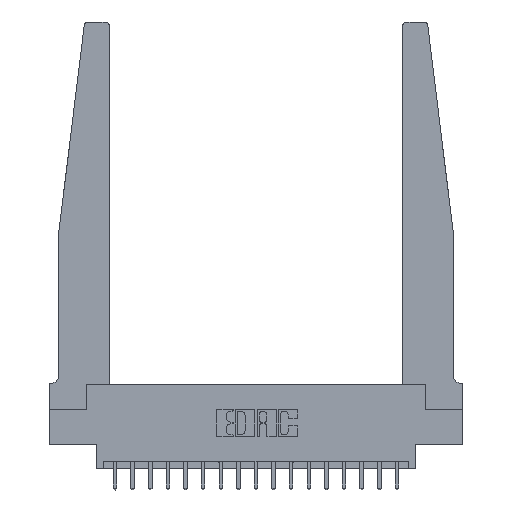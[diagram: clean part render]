
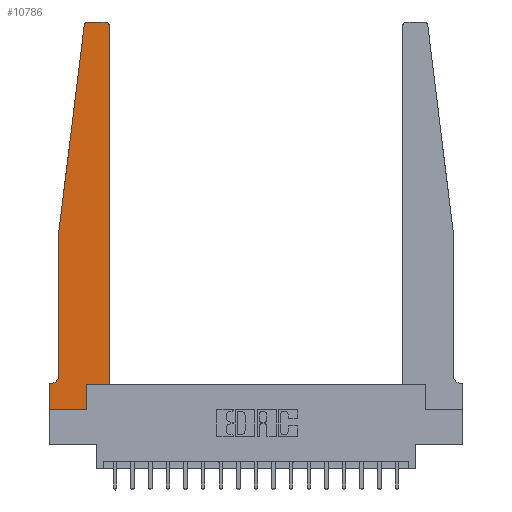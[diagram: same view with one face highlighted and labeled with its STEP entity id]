
A CAD part, top view. The second image highlights one B-rep face of the part: STEP entity #10786.
In plain terms, the highlighted planar face has unit normal (0, 0, 1).
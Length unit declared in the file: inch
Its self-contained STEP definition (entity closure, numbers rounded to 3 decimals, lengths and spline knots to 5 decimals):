
#241 = EDGE_LOOP ( 'NONE', ( #7035, #4532, #2124, #3526, #17690, #8362, #7647, #2840, #19340, #8499, #999, #5198 ) ) ;
#347 = EDGE_CURVE ( 'NONE', #17558, #3035, #9736, .T. ) ;
#404 = VERTEX_POINT ( 'NONE', #5014 ) ;
#543 = DIRECTION ( 'NONE',  ( 1., 0., 0. ) ) ;
#586 = CARTESIAN_POINT ( 'NONE',  ( 0., 0., 0.37 ) ) ;
#904 = FACE_OUTER_BOUND ( 'NONE', #241, .T. ) ;
#978 = EDGE_CURVE ( 'NONE', #2841, #15863, #7843, .T. ) ;
#999 = ORIENTED_EDGE ( 'NONE', *, *, #6301, .T. ) ;
#1581 = AXIS2_PLACEMENT_3D ( 'NONE', #8735, #19105, #10205 ) ;
#1583 = CARTESIAN_POINT ( 'NONE',  ( 0.065, 1.25, 0.37 ) ) ;
#1772 = VECTOR ( 'NONE', #13612, 39.37008 ) ;
#1785 = VERTEX_POINT ( 'NONE', #15458 ) ;
#2094 = LINE ( 'NONE', #16965, #10116 ) ;
#2124 = ORIENTED_EDGE ( 'NONE', *, *, #347, .T. ) ;
#2294 = DIRECTION ( 'NONE',  ( 1., 0., 0. ) ) ;
#2455 = CARTESIAN_POINT ( 'NONE',  ( 0.395, 2.75, 0.37 ) ) ;
#2758 = LINE ( 'NONE', #3187, #1772 ) ;
#2840 = ORIENTED_EDGE ( 'NONE', *, *, #11048, .T. ) ;
#2841 = VERTEX_POINT ( 'NONE', #3572 ) ;
#3035 = VERTEX_POINT ( 'NONE', #1583 ) ;
#3039 = VECTOR ( 'NONE', #10518, 39.37008 ) ;
#3187 = CARTESIAN_POINT ( 'NONE',  ( 0.2605, 0.18, 0.37 ) ) ;
#3188 = PLANE ( 'NONE',  #17655 ) ;
#3526 = ORIENTED_EDGE ( 'NONE', *, *, #4661, .T. ) ;
#3572 = CARTESIAN_POINT ( 'NONE',  ( 0.065, 0.2375, 0.37 ) ) ;
#3603 = CARTESIAN_POINT ( 'NONE',  ( 0.425, 0.18, 0.37 ) ) ;
#4035 = CARTESIAN_POINT ( 'NONE',  ( 0., 0.1875, 0.37 ) ) ;
#4042 = CARTESIAN_POINT ( 'NONE',  ( 0., 0., 0.37 ) ) ;
#4532 = ORIENTED_EDGE ( 'NONE', *, *, #7488, .T. ) ;
#4661 = EDGE_CURVE ( 'NONE', #3035, #2841, #2094, .T. ) ;
#4680 = DIRECTION ( 'NONE',  ( 1., 0., 0. ) ) ;
#4804 = DIRECTION ( 'NONE',  ( -1., 0., 0. ) ) ;
#4996 = AXIS2_PLACEMENT_3D ( 'NONE', #14276, #5330, #15735 ) ;
#5014 = CARTESIAN_POINT ( 'NONE',  ( 0.27653, 2.75, 0.37 ) ) ;
#5054 = CARTESIAN_POINT ( 'NONE',  ( 0.425, 2.72, 0.37 ) ) ;
#5198 = ORIENTED_EDGE ( 'NONE', *, *, #10565, .T. ) ;
#5330 = DIRECTION ( 'NONE',  ( 0., 0., 1. ) ) ;
#5398 = VERTEX_POINT ( 'NONE', #2455 ) ;
#5436 = DIRECTION ( 'NONE',  ( 0., 1., 0. ) ) ;
#5457 = CARTESIAN_POINT ( 'NONE',  ( 0.015, 0.1875, 0.37 ) ) ;
#5622 = EDGE_CURVE ( 'NONE', #5398, #404, #7051, .T. ) ;
#5712 = CARTESIAN_POINT ( 'NONE',  ( 0., 0., 0.37 ) ) ;
#6301 = EDGE_CURVE ( 'NONE', #15176, #11398, #15571, .T. ) ;
#6948 = CARTESIAN_POINT ( 'NONE',  ( 0.425, 0.18, 0.37 ) ) ;
#7035 = ORIENTED_EDGE ( 'NONE', *, *, #5622, .T. ) ;
#7051 = LINE ( 'NONE', #7473, #3039 ) ;
#7473 = CARTESIAN_POINT ( 'NONE',  ( 0.25, 2.75, 0.37 ) ) ;
#7488 = EDGE_CURVE ( 'NONE', #404, #17558, #16716, .T. ) ;
#7647 = ORIENTED_EDGE ( 'NONE', *, *, #11857, .T. ) ;
#7789 = CARTESIAN_POINT ( 'NONE',  ( 0.065, 0.1875, 0.37 ) ) ;
#7843 = CIRCLE ( 'NONE', #8001, 0.05 ) ;
#7969 = LINE ( 'NONE', #4042, #14457 ) ;
#8001 = AXIS2_PLACEMENT_3D ( 'NONE', #10732, #13978, #12918 ) ;
#8103 = DIRECTION ( 'NONE',  ( 0., -1., 0. ) ) ;
#8171 = VERTEX_POINT ( 'NONE', #5712 ) ;
#8237 = LINE ( 'NONE', #586, #12130 ) ;
#8362 = ORIENTED_EDGE ( 'NONE', *, *, #12185, .T. ) ;
#8499 = ORIENTED_EDGE ( 'NONE', *, *, #11619, .T. ) ;
#8735 = CARTESIAN_POINT ( 'NONE',  ( 0.395, 2.72, 0.37 ) ) ;
#8889 = CARTESIAN_POINT ( 'NONE',  ( 0.065, 1.25, 0.37 ) ) ;
#9642 = DIRECTION ( 'NONE',  ( -0.122, -0.992, 0. ) ) ;
#9736 = LINE ( 'NONE', #8889, #17624 ) ;
#10116 = VECTOR ( 'NONE', #8103, 39.37008 ) ;
#10205 = DIRECTION ( 'NONE',  ( 1., 0., 0. ) ) ;
#10518 = DIRECTION ( 'NONE',  ( -1., 0., 0. ) ) ;
#10565 = EDGE_CURVE ( 'NONE', #11398, #5398, #16576, .T. ) ;
#10732 = CARTESIAN_POINT ( 'NONE',  ( 0.015, 0.2375, 0.37 ) ) ;
#10742 = VECTOR ( 'NONE', #543, 39.37008 ) ;
#10786 = ADVANCED_FACE ( 'NONE', ( #904 ), #3188, .T. ) ;
#11048 = EDGE_CURVE ( 'NONE', #8171, #17473, #8237, .T. ) ;
#11210 = LINE ( 'NONE', #3603, #10742 ) ;
#11398 = VERTEX_POINT ( 'NONE', #5054 ) ;
#11619 = EDGE_CURVE ( 'NONE', #1785, #15176, #11210, .T. ) ;
#11658 = VECTOR ( 'NONE', #5436, 39.37008 ) ;
#11857 = EDGE_CURVE ( 'NONE', #13692, #8171, #7969, .T. ) ;
#12100 = CARTESIAN_POINT ( 'NONE',  ( 0., 0.1875, 0.37 ) ) ;
#12129 = EDGE_CURVE ( 'NONE', #17473, #1785, #2758, .T. ) ;
#12130 = VECTOR ( 'NONE', #2294, 39.37008 ) ;
#12185 = EDGE_CURVE ( 'NONE', #15863, #13692, #12824, .T. ) ;
#12328 = VECTOR ( 'NONE', #4804, 39.37008 ) ;
#12824 = LINE ( 'NONE', #7789, #12328 ) ;
#12882 = CARTESIAN_POINT ( 'NONE',  ( 0.425, 0.18, 0.37 ) ) ;
#12918 = DIRECTION ( 'NONE',  ( -1., 0., 0. ) ) ;
#13612 = DIRECTION ( 'NONE',  ( 0., 1., 0. ) ) ;
#13613 = DIRECTION ( 'NONE',  ( 0., 0., 1. ) ) ;
#13692 = VERTEX_POINT ( 'NONE', #4035 ) ;
#13978 = DIRECTION ( 'NONE',  ( 0., 0., -1. ) ) ;
#14276 = CARTESIAN_POINT ( 'NONE',  ( 0.27653, 2.72, 0.37 ) ) ;
#14457 = VECTOR ( 'NONE', #14545, 39.37008 ) ;
#14545 = DIRECTION ( 'NONE',  ( 0., -1., 0. ) ) ;
#15176 = VERTEX_POINT ( 'NONE', #6948 ) ;
#15458 = CARTESIAN_POINT ( 'NONE',  ( 0.2605, 0.18, 0.37 ) ) ;
#15571 = LINE ( 'NONE', #12882, #11658 ) ;
#15735 = DIRECTION ( 'NONE',  ( 1., 0., 0. ) ) ;
#15863 = VERTEX_POINT ( 'NONE', #5457 ) ;
#16315 = CARTESIAN_POINT ( 'NONE',  ( 0.2605, 0., 0.37 ) ) ;
#16576 = CIRCLE ( 'NONE', #1581, 0.03 ) ;
#16716 = CIRCLE ( 'NONE', #4996, 0.03 ) ;
#16965 = CARTESIAN_POINT ( 'NONE',  ( 0.065, 1.25, 0.37 ) ) ;
#17473 = VERTEX_POINT ( 'NONE', #16315 ) ;
#17558 = VERTEX_POINT ( 'NONE', #17931 ) ;
#17624 = VECTOR ( 'NONE', #9642, 39.37008 ) ;
#17655 = AXIS2_PLACEMENT_3D ( 'NONE', #12100, #13613, #4680 ) ;
#17690 = ORIENTED_EDGE ( 'NONE', *, *, #978, .T. ) ;
#17931 = CARTESIAN_POINT ( 'NONE',  ( 0.24675, 2.72367, 0.37 ) ) ;
#19105 = DIRECTION ( 'NONE',  ( 0., 0., 1. ) ) ;
#19340 = ORIENTED_EDGE ( 'NONE', *, *, #12129, .T. ) ;
